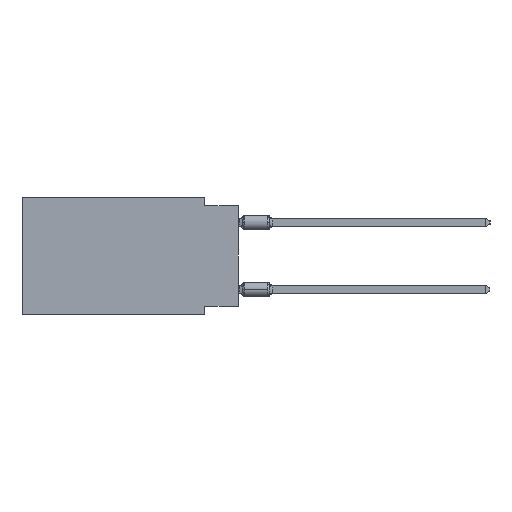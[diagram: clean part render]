
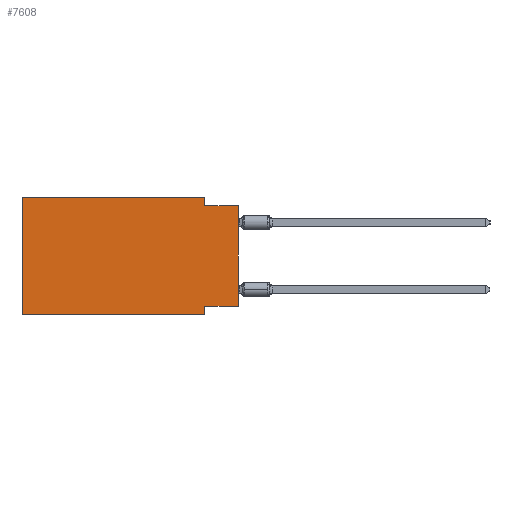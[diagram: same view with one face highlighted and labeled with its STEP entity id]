
A CAD part, left-side view. The second image highlights one B-rep face of the part: STEP entity #7608.
In plain terms, the highlighted planar face has unit normal (-1, 0, 0).
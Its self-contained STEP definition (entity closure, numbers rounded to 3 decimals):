
#17 = CARTESIAN_POINT ( 'NONE',  ( 0., 16.383, 0. ) ) ;
#382 = ORIENTED_EDGE ( 'NONE', *, *, #20408, .F. ) ;
#622 = EDGE_CURVE ( 'NONE', #5679, #18901, #6130, .T. ) ;
#2274 = PLANE ( 'NONE',  #15841 ) ;
#2440 = ORIENTED_EDGE ( 'NONE', *, *, #3908, .F. ) ;
#2706 = VERTEX_POINT ( 'NONE', #28302 ) ;
#3304 = EDGE_CURVE ( 'NONE', #5679, #14345, #33613, .T. ) ;
#3908 = EDGE_CURVE ( 'NONE', #20139, #13505, #19625, .T. ) ;
#4941 = CARTESIAN_POINT ( 'NONE',  ( 0., 2.54, 0. ) ) ;
#5679 = VERTEX_POINT ( 'NONE', #32735 ) ;
#6130 = LINE ( 'NONE', #24096, #14574 ) ;
#6184 = VECTOR ( 'NONE', #11818, 1000. ) ;
#6592 = DIRECTION ( 'NONE',  ( 0., -1., 0. ) ) ;
#7608 = ADVANCED_FACE ( 'NONE', ( #34939 ), #2274, .F. ) ;
#7939 = EDGE_CURVE ( 'NONE', #33932, #37828, #9405, .T. ) ;
#9174 = DIRECTION ( 'NONE',  ( 0., 0., -1. ) ) ;
#9405 = LINE ( 'NONE', #26621, #31952 ) ;
#10500 = EDGE_CURVE ( 'NONE', #13505, #18901, #34990, .T. ) ;
#11683 = CARTESIAN_POINT ( 'NONE',  ( 0., 0., -0.635 ) ) ;
#11818 = DIRECTION ( 'NONE',  ( 0., 0., 1. ) ) ;
#13505 = VERTEX_POINT ( 'NONE', #30430 ) ;
#13652 = ORIENTED_EDGE ( 'NONE', *, *, #32748, .F. ) ;
#13825 = DIRECTION ( 'NONE',  ( 0., 0., -1. ) ) ;
#14345 = VERTEX_POINT ( 'NONE', #17569 ) ;
#14574 = VECTOR ( 'NONE', #35505, 1000. ) ;
#15841 = AXIS2_PLACEMENT_3D ( 'NONE', #16769, #20242, #22766 ) ;
#16754 = ORIENTED_EDGE ( 'NONE', *, *, #7939, .T. ) ;
#16769 = CARTESIAN_POINT ( 'NONE',  ( 0., 16.383, 0. ) ) ;
#17569 = CARTESIAN_POINT ( 'NONE',  ( 0., 2.54, -8.255 ) ) ;
#17960 = DIRECTION ( 'NONE',  ( 0., 1., 0. ) ) ;
#18901 = VERTEX_POINT ( 'NONE', #11683 ) ;
#19625 = LINE ( 'NONE', #4941, #28004 ) ;
#20139 = VERTEX_POINT ( 'NONE', #25943 ) ;
#20242 = DIRECTION ( 'NONE',  ( 1., 0., 0. ) ) ;
#20408 = EDGE_CURVE ( 'NONE', #2706, #20139, #21831, .T. ) ;
#21831 = LINE ( 'NONE', #33637, #35440 ) ;
#22332 = ORIENTED_EDGE ( 'NONE', *, *, #10500, .F. ) ;
#22766 = DIRECTION ( 'NONE',  ( 0., 0., -1. ) ) ;
#23739 = ORIENTED_EDGE ( 'NONE', *, *, #622, .T. ) ;
#24096 = CARTESIAN_POINT ( 'NONE',  ( 0., 0., 0. ) ) ;
#24279 = DIRECTION ( 'NONE',  ( 0., -1., 0. ) ) ;
#25266 = EDGE_CURVE ( 'NONE', #14345, #37828, #35076, .T. ) ;
#25779 = ORIENTED_EDGE ( 'NONE', *, *, #3304, .F. ) ;
#25943 = CARTESIAN_POINT ( 'NONE',  ( 0., 2.54, 0. ) ) ;
#25992 = CARTESIAN_POINT ( 'NONE',  ( 0., 2.54, -8.89 ) ) ;
#26396 = CARTESIAN_POINT ( 'NONE',  ( 0., 2.54, -8.89 ) ) ;
#26621 = CARTESIAN_POINT ( 'NONE',  ( 0., 16.383, -8.89 ) ) ;
#27035 = VECTOR ( 'NONE', #9174, 1000. ) ;
#28004 = VECTOR ( 'NONE', #13825, 1000. ) ;
#28059 = EDGE_LOOP ( 'NONE', ( #23739, #22332, #2440, #382, #13652, #16754, #38059, #25779 ) ) ;
#28302 = CARTESIAN_POINT ( 'NONE',  ( 0., 16.383, 0. ) ) ;
#29887 = VECTOR ( 'NONE', #17960, 1000. ) ;
#29993 = CARTESIAN_POINT ( 'NONE',  ( 0., 16.383, -8.89 ) ) ;
#30430 = CARTESIAN_POINT ( 'NONE',  ( 0., 2.54, -0.635 ) ) ;
#31952 = VECTOR ( 'NONE', #24279, 1000. ) ;
#32103 = DIRECTION ( 'NONE',  ( 0., -1., 0. ) ) ;
#32120 = VECTOR ( 'NONE', #32103, 1000. ) ;
#32706 = LINE ( 'NONE', #17, #6184 ) ;
#32735 = CARTESIAN_POINT ( 'NONE',  ( 0., 0., -8.255 ) ) ;
#32748 = EDGE_CURVE ( 'NONE', #33932, #2706, #32706, .T. ) ;
#33436 = CARTESIAN_POINT ( 'NONE',  ( 0., 0., -8.255 ) ) ;
#33613 = LINE ( 'NONE', #33436, #29887 ) ;
#33637 = CARTESIAN_POINT ( 'NONE',  ( 0., 16.383, 0. ) ) ;
#33932 = VERTEX_POINT ( 'NONE', #29993 ) ;
#34939 = FACE_OUTER_BOUND ( 'NONE', #28059, .T. ) ;
#34990 = LINE ( 'NONE', #35187, #32120 ) ;
#35076 = LINE ( 'NONE', #25992, #27035 ) ;
#35187 = CARTESIAN_POINT ( 'NONE',  ( 0., 0., -0.635 ) ) ;
#35440 = VECTOR ( 'NONE', #6592, 1000. ) ;
#35505 = DIRECTION ( 'NONE',  ( 0., 0., 1. ) ) ;
#37828 = VERTEX_POINT ( 'NONE', #26396 ) ;
#38059 = ORIENTED_EDGE ( 'NONE', *, *, #25266, .F. ) ;
